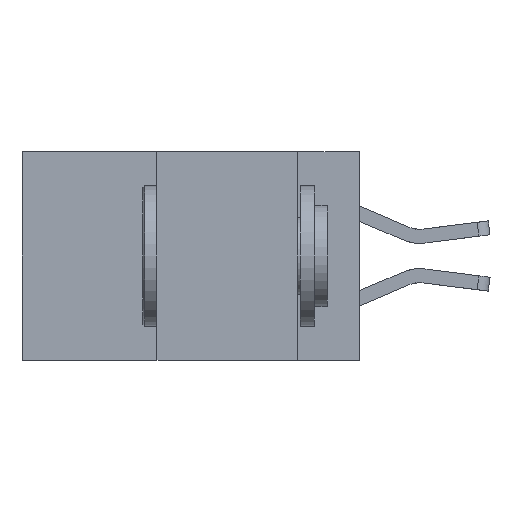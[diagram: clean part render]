
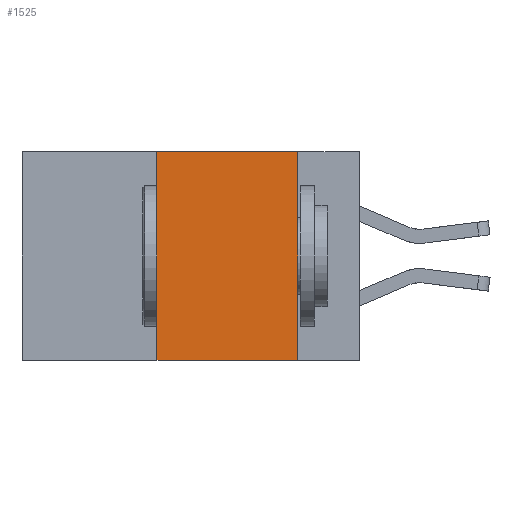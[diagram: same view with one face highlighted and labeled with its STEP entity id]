
A CAD part, left-side view. The second image highlights one B-rep face of the part: STEP entity #1525.
In plain terms, the highlighted planar face has unit normal (-1, 0, 0).
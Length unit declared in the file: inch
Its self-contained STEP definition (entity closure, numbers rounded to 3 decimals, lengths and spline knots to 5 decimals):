
#44 = VECTOR ( 'NONE', #11551, 39.37008 ) ;
#187 = FACE_OUTER_BOUND ( 'NONE', #7029, .T. ) ;
#386 = LINE ( 'NONE', #9599, #44 ) ;
#1103 = ORIENTED_EDGE ( 'NONE', *, *, #9669, .T. ) ;
#1353 = LINE ( 'NONE', #6080, #8576 ) ;
#1360 = CARTESIAN_POINT ( 'NONE',  ( 0., 0.11, -0.37 ) ) ;
#1525 = ADVANCED_FACE ( 'NONE', ( #187 ), #3523, .F. ) ;
#1804 = DIRECTION ( 'NONE',  ( 1., 0., 0. ) ) ;
#1883 = VECTOR ( 'NONE', #10147, 39.37008 ) ;
#2051 = LINE ( 'NONE', #8083, #1883 ) ;
#2068 = VERTEX_POINT ( 'NONE', #5675 ) ;
#3012 = CARTESIAN_POINT ( 'NONE',  ( 0., 0.36, -0.37 ) ) ;
#3138 = VECTOR ( 'NONE', #13264, 39.37008 ) ;
#3259 = ORIENTED_EDGE ( 'NONE', *, *, #11647, .F. ) ;
#3523 = PLANE ( 'NONE',  #11513 ) ;
#3725 = DIRECTION ( 'NONE',  ( 0., 0., -1. ) ) ;
#3832 = ORIENTED_EDGE ( 'NONE', *, *, #9404, .F. ) ;
#4425 = VERTEX_POINT ( 'NONE', #7195 ) ;
#5675 = CARTESIAN_POINT ( 'NONE',  ( 0., 0.11, 0. ) ) ;
#6080 = CARTESIAN_POINT ( 'NONE',  ( 0., 0.11, 0. ) ) ;
#6221 = CARTESIAN_POINT ( 'NONE',  ( 0., 0.36, 0. ) ) ;
#6234 = VERTEX_POINT ( 'NONE', #3012 ) ;
#6358 = LINE ( 'NONE', #6221, #3138 ) ;
#7029 = EDGE_LOOP ( 'NONE', ( #3832, #12427, #3259, #1103 ) ) ;
#7195 = CARTESIAN_POINT ( 'NONE',  ( 0., 0.36, 0. ) ) ;
#7981 = EDGE_CURVE ( 'NONE', #4425, #2068, #2051, .T. ) ;
#8083 = CARTESIAN_POINT ( 'NONE',  ( 0., 0.6, 0. ) ) ;
#8162 = VERTEX_POINT ( 'NONE', #1360 ) ;
#8573 = DIRECTION ( 'NONE',  ( 0., 0., -1. ) ) ;
#8576 = VECTOR ( 'NONE', #8573, 39.37008 ) ;
#9404 = EDGE_CURVE ( 'NONE', #2068, #8162, #1353, .T. ) ;
#9599 = CARTESIAN_POINT ( 'NONE',  ( 0., 0.6, -0.37 ) ) ;
#9669 = EDGE_CURVE ( 'NONE', #6234, #8162, #386, .T. ) ;
#10147 = DIRECTION ( 'NONE',  ( 0., -1., 0. ) ) ;
#10680 = CARTESIAN_POINT ( 'NONE',  ( 0., 0.6, 0. ) ) ;
#11513 = AXIS2_PLACEMENT_3D ( 'NONE', #10680, #1804, #3725 ) ;
#11551 = DIRECTION ( 'NONE',  ( 0., -1., 0. ) ) ;
#11647 = EDGE_CURVE ( 'NONE', #6234, #4425, #6358, .T. ) ;
#12427 = ORIENTED_EDGE ( 'NONE', *, *, #7981, .F. ) ;
#13264 = DIRECTION ( 'NONE',  ( 0., 0., 1. ) ) ;
